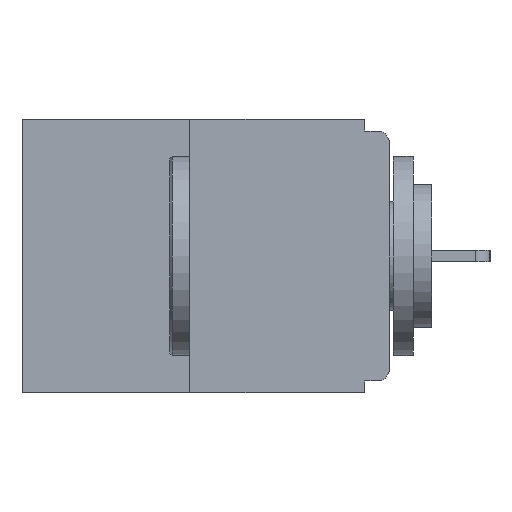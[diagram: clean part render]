
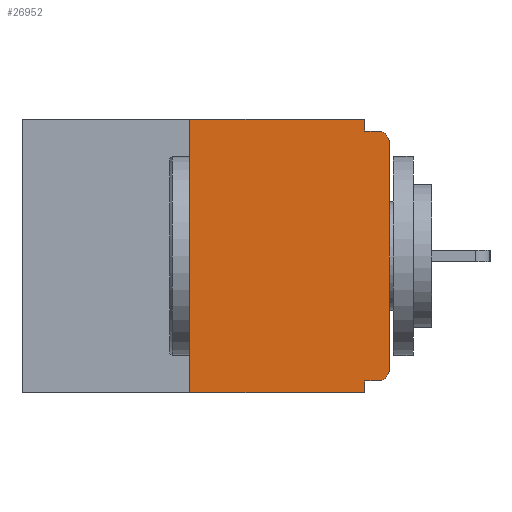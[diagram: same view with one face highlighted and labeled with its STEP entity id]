
A CAD part, left-side view. The second image highlights one B-rep face of the part: STEP entity #26952.
In plain terms, the highlighted planar face has unit normal (-1, 0, 0).
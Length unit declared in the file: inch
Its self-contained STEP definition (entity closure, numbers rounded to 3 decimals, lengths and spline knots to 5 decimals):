
#28 = CARTESIAN_POINT ( 'NONE',  ( 0., 0.031, -0.343 ) ) ;
#98 = VECTOR ( 'NONE', #17985, 39.37008 ) ;
#105 = LINE ( 'NONE', #8530, #24707 ) ;
#853 = AXIS2_PLACEMENT_3D ( 'NONE', #3005, #19732, #22370 ) ;
#1870 = CARTESIAN_POINT ( 'NONE',  ( 0., 0.25, 0. ) ) ;
#2034 = VERTEX_POINT ( 'NONE', #13328 ) ;
#2065 = ORIENTED_EDGE ( 'NONE', *, *, #9991, .T. ) ;
#2572 = CARTESIAN_POINT ( 'NONE',  ( 0., 0.031, -0.328 ) ) ;
#2929 = LINE ( 'NONE', #24223, #98 ) ;
#3005 = CARTESIAN_POINT ( 'NONE',  ( 0., 0.015, -0.03 ) ) ;
#3127 = EDGE_CURVE ( 'NONE', #2034, #17266, #105, .T. ) ;
#3698 = CARTESIAN_POINT ( 'NONE',  ( 0., 0., -0.015 ) ) ;
#3864 = VERTEX_POINT ( 'NONE', #19955 ) ;
#4210 = LINE ( 'NONE', #1870, #12446 ) ;
#4546 = ORIENTED_EDGE ( 'NONE', *, *, #23687, .F. ) ;
#4585 = ORIENTED_EDGE ( 'NONE', *, *, #12214, .T. ) ;
#4977 = CIRCLE ( 'NONE', #5409, 0.015 ) ;
#5003 = VECTOR ( 'NONE', #24611, 39.37008 ) ;
#5198 = CARTESIAN_POINT ( 'NONE',  ( 0., 0., -0.03 ) ) ;
#5409 = AXIS2_PLACEMENT_3D ( 'NONE', #14137, #13865, #26891 ) ;
#6019 = CARTESIAN_POINT ( 'NONE',  ( 0., 0.46, -0.343 ) ) ;
#6107 = EDGE_CURVE ( 'NONE', #10688, #3864, #4977, .T. ) ;
#6590 = CARTESIAN_POINT ( 'NONE',  ( 0., 0.015, -0.015 ) ) ;
#6702 = ORIENTED_EDGE ( 'NONE', *, *, #19959, .F. ) ;
#7131 = VERTEX_POINT ( 'NONE', #2572 ) ;
#7311 = LINE ( 'NONE', #16895, #21879 ) ;
#7621 = VECTOR ( 'NONE', #14850, 39.37008 ) ;
#7725 = LINE ( 'NONE', #16156, #5003 ) ;
#8226 = LINE ( 'NONE', #6019, #7621 ) ;
#8246 = LINE ( 'NONE', #3698, #11735 ) ;
#8530 = CARTESIAN_POINT ( 'NONE',  ( 0., 0.031, 0. ) ) ;
#8596 = CARTESIAN_POINT ( 'NONE',  ( 0., 0.46, 0. ) ) ;
#9634 = DIRECTION ( 'NONE',  ( 0., -1., 0. ) ) ;
#9991 = EDGE_CURVE ( 'NONE', #26389, #12914, #10118, .T. ) ;
#10118 = CIRCLE ( 'NONE', #853, 0.015 ) ;
#10395 = ORIENTED_EDGE ( 'NONE', *, *, #13398, .T. ) ;
#10688 = VERTEX_POINT ( 'NONE', #21868 ) ;
#11735 = VECTOR ( 'NONE', #12109, 39.37008 ) ;
#12109 = DIRECTION ( 'NONE',  ( 0., -1., 0. ) ) ;
#12119 = ORIENTED_EDGE ( 'NONE', *, *, #3127, .F. ) ;
#12214 = EDGE_CURVE ( 'NONE', #3864, #26389, #2929, .T. ) ;
#12446 = VECTOR ( 'NONE', #14430, 39.37008 ) ;
#12700 = DIRECTION ( 'NONE',  ( 1., 0., 0. ) ) ;
#12914 = VERTEX_POINT ( 'NONE', #6590 ) ;
#13328 = CARTESIAN_POINT ( 'NONE',  ( 0., 0.031, 0. ) ) ;
#13336 = EDGE_CURVE ( 'NONE', #16885, #15587, #4210, .T. ) ;
#13398 = EDGE_CURVE ( 'NONE', #16885, #17105, #8226, .T. ) ;
#13629 = CARTESIAN_POINT ( 'NONE',  ( 0., 0.46, 0. ) ) ;
#13865 = DIRECTION ( 'NONE',  ( -1., 0., 0. ) ) ;
#14117 = EDGE_CURVE ( 'NONE', #10688, #7131, #7725, .T. ) ;
#14137 = CARTESIAN_POINT ( 'NONE',  ( 0., 0.015, -0.313 ) ) ;
#14430 = DIRECTION ( 'NONE',  ( 0., 0., 1. ) ) ;
#14850 = DIRECTION ( 'NONE',  ( 0., -1., 0. ) ) ;
#15587 = VERTEX_POINT ( 'NONE', #22000 ) ;
#16156 = CARTESIAN_POINT ( 'NONE',  ( 0., 0., -0.328 ) ) ;
#16885 = VERTEX_POINT ( 'NONE', #19019 ) ;
#16895 = CARTESIAN_POINT ( 'NONE',  ( 0., 0.031, -0.343 ) ) ;
#16962 = DIRECTION ( 'NONE',  ( 0., 0., -1. ) ) ;
#17105 = VERTEX_POINT ( 'NONE', #28 ) ;
#17266 = VERTEX_POINT ( 'NONE', #23813 ) ;
#17683 = DIRECTION ( 'NONE',  ( 0., 0., -1. ) ) ;
#17985 = DIRECTION ( 'NONE',  ( 0., 0., 1. ) ) ;
#18953 = PLANE ( 'NONE',  #18958 ) ;
#18958 = AXIS2_PLACEMENT_3D ( 'NONE', #8596, #12700, #20914 ) ;
#19019 = CARTESIAN_POINT ( 'NONE',  ( 0., 0.25, -0.343 ) ) ;
#19390 = ORIENTED_EDGE ( 'NONE', *, *, #13336, .F. ) ;
#19732 = DIRECTION ( 'NONE',  ( -1., 0., 0. ) ) ;
#19955 = CARTESIAN_POINT ( 'NONE',  ( 0., 0., -0.313 ) ) ;
#19959 = EDGE_CURVE ( 'NONE', #7131, #17105, #7311, .T. ) ;
#20914 = DIRECTION ( 'NONE',  ( 0., 0., -1. ) ) ;
#21868 = CARTESIAN_POINT ( 'NONE',  ( 0., 0.015, -0.328 ) ) ;
#21879 = VECTOR ( 'NONE', #17683, 39.37008 ) ;
#22000 = CARTESIAN_POINT ( 'NONE',  ( 0., 0.25, 0. ) ) ;
#22370 = DIRECTION ( 'NONE',  ( 0., 0., -1. ) ) ;
#22573 = ORIENTED_EDGE ( 'NONE', *, *, #14117, .F. ) ;
#23630 = EDGE_CURVE ( 'NONE', #15587, #2034, #24178, .T. ) ;
#23687 = EDGE_CURVE ( 'NONE', #17266, #12914, #8246, .T. ) ;
#23813 = CARTESIAN_POINT ( 'NONE',  ( 0., 0.031, -0.015 ) ) ;
#23852 = ORIENTED_EDGE ( 'NONE', *, *, #23630, .F. ) ;
#24178 = LINE ( 'NONE', #13629, #25025 ) ;
#24223 = CARTESIAN_POINT ( 'NONE',  ( 0., 0., 0. ) ) ;
#24611 = DIRECTION ( 'NONE',  ( 0., 1., 0. ) ) ;
#24707 = VECTOR ( 'NONE', #16962, 39.37008 ) ;
#25025 = VECTOR ( 'NONE', #9634, 39.37008 ) ;
#25169 = ORIENTED_EDGE ( 'NONE', *, *, #6107, .T. ) ;
#25435 = EDGE_LOOP ( 'NONE', ( #23852, #19390, #10395, #6702, #22573, #25169, #4585, #2065, #4546, #12119 ) ) ;
#25475 = FACE_OUTER_BOUND ( 'NONE', #25435, .T. ) ;
#26389 = VERTEX_POINT ( 'NONE', #5198 ) ;
#26891 = DIRECTION ( 'NONE',  ( 0., 0., -1. ) ) ;
#26952 = ADVANCED_FACE ( 'NONE', ( #25475 ), #18953, .F. ) ;
